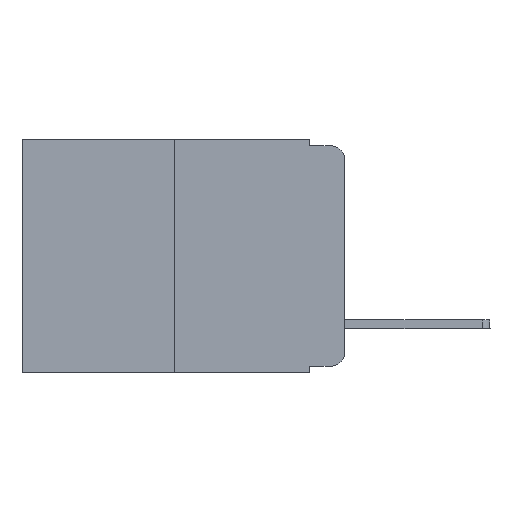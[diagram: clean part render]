
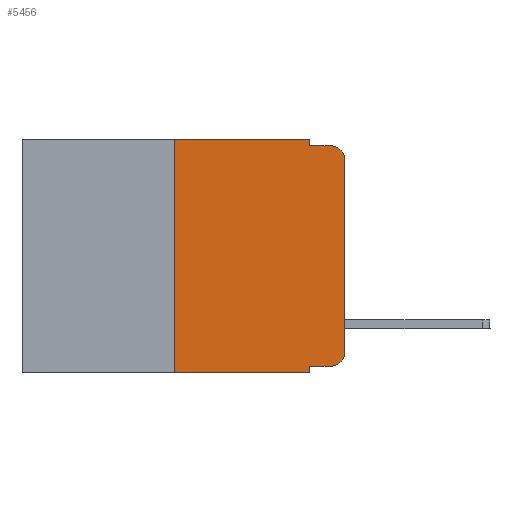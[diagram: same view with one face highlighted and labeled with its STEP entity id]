
A CAD part, left-side view. The second image highlights one B-rep face of the part: STEP entity #5456.
In plain terms, the highlighted planar face has unit normal (-1, 0, 0).
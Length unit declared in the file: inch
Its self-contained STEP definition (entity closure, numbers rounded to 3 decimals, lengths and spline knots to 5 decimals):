
#315 = CIRCLE ( 'NONE', #18076, 0.02 ) ;
#862 = CARTESIAN_POINT ( 'NONE',  ( 0., 0.473, 0. ) ) ;
#989 = DIRECTION ( 'NONE',  ( 0., -1., 0. ) ) ;
#1194 = LINE ( 'NONE', #10597, #11371 ) ;
#1485 = CARTESIAN_POINT ( 'NONE',  ( 0., 0.051, -0.333 ) ) ;
#1515 = DIRECTION ( 'NONE',  ( 0., 0., -1. ) ) ;
#1546 = VERTEX_POINT ( 'NONE', #13739 ) ;
#1560 = EDGE_CURVE ( 'NONE', #16669, #8262, #315, .T. ) ;
#1661 = VECTOR ( 'NONE', #1515, 39.37008 ) ;
#2155 = DIRECTION ( 'NONE',  ( 0., 0., -1. ) ) ;
#2189 = LINE ( 'NONE', #8463, #17527 ) ;
#2337 = DIRECTION ( 'NONE',  ( 0., 0., 1. ) ) ;
#2345 = EDGE_CURVE ( 'NONE', #1546, #4240, #16555, .T. ) ;
#2663 = EDGE_CURVE ( 'NONE', #6638, #1546, #8502, .T. ) ;
#3662 = CARTESIAN_POINT ( 'NONE',  ( 0., 0.25, 0. ) ) ;
#3822 = VECTOR ( 'NONE', #6338, 39.37008 ) ;
#3948 = ORIENTED_EDGE ( 'NONE', *, *, #2663, .F. ) ;
#4146 = EDGE_CURVE ( 'NONE', #17577, #16669, #2189, .T. ) ;
#4240 = VERTEX_POINT ( 'NONE', #6729 ) ;
#4476 = ORIENTED_EDGE ( 'NONE', *, *, #2345, .F. ) ;
#4644 = DIRECTION ( 'NONE',  ( 0., 0., 1. ) ) ;
#4836 = CARTESIAN_POINT ( 'NONE',  ( 0., 0.02, -0.01 ) ) ;
#4840 = CARTESIAN_POINT ( 'NONE',  ( 0., 0.473, 0. ) ) ;
#5456 = ADVANCED_FACE ( 'NONE', ( #16043 ), #9878, .F. ) ;
#5528 = LINE ( 'NONE', #3662, #7633 ) ;
#5599 = LINE ( 'NONE', #14200, #12645 ) ;
#5981 = CARTESIAN_POINT ( 'NONE',  ( 0., 0.051, 0. ) ) ;
#6224 = ORIENTED_EDGE ( 'NONE', *, *, #1560, .T. ) ;
#6271 = VERTEX_POINT ( 'NONE', #4836 ) ;
#6338 = DIRECTION ( 'NONE',  ( 0., -1., 0. ) ) ;
#6380 = CARTESIAN_POINT ( 'NONE',  ( 0., 0.051, -0.01 ) ) ;
#6416 = ORIENTED_EDGE ( 'NONE', *, *, #13997, .F. ) ;
#6638 = VERTEX_POINT ( 'NONE', #11368 ) ;
#6729 = CARTESIAN_POINT ( 'NONE',  ( 0., 0.051, -0.01 ) ) ;
#6916 = ORIENTED_EDGE ( 'NONE', *, *, #14733, .T. ) ;
#7131 = AXIS2_PLACEMENT_3D ( 'NONE', #862, #8509, #12958 ) ;
#7633 = VECTOR ( 'NONE', #2337, 39.37008 ) ;
#7795 = ORIENTED_EDGE ( 'NONE', *, *, #16438, .F. ) ;
#8019 = DIRECTION ( 'NONE',  ( -1., 0., 0. ) ) ;
#8103 = VERTEX_POINT ( 'NONE', #12424 ) ;
#8156 = CARTESIAN_POINT ( 'NONE',  ( 0., 0.02, -0.03 ) ) ;
#8262 = VERTEX_POINT ( 'NONE', #16104 ) ;
#8365 = LINE ( 'NONE', #6380, #18997 ) ;
#8463 = CARTESIAN_POINT ( 'NONE',  ( 0., 0.051, -0.333 ) ) ;
#8502 = LINE ( 'NONE', #4840, #3822 ) ;
#8509 = DIRECTION ( 'NONE',  ( 1., 0., 0. ) ) ;
#8674 = ORIENTED_EDGE ( 'NONE', *, *, #15822, .F. ) ;
#9121 = CARTESIAN_POINT ( 'NONE',  ( 0., 0.051, -0.343 ) ) ;
#9541 = VECTOR ( 'NONE', #989, 39.37008 ) ;
#9673 = AXIS2_PLACEMENT_3D ( 'NONE', #8156, #8019, #2155 ) ;
#9878 = PLANE ( 'NONE',  #7131 ) ;
#10597 = CARTESIAN_POINT ( 'NONE',  ( 0., 0., 0. ) ) ;
#10675 = DIRECTION ( 'NONE',  ( -1., 0., 0. ) ) ;
#10779 = EDGE_CURVE ( 'NONE', #8103, #6271, #11742, .T. ) ;
#11368 = CARTESIAN_POINT ( 'NONE',  ( 0., 0.25, 0. ) ) ;
#11371 = VECTOR ( 'NONE', #4644, 39.37008 ) ;
#11389 = CARTESIAN_POINT ( 'NONE',  ( 0., 0.02, -0.333 ) ) ;
#11742 = CIRCLE ( 'NONE', #9673, 0.02 ) ;
#11764 = EDGE_CURVE ( 'NONE', #17729, #12233, #15708, .T. ) ;
#11970 = DIRECTION ( 'NONE',  ( 0., -1., 0. ) ) ;
#12233 = VERTEX_POINT ( 'NONE', #9121 ) ;
#12424 = CARTESIAN_POINT ( 'NONE',  ( 0., 0., -0.03 ) ) ;
#12645 = VECTOR ( 'NONE', #14275, 39.37008 ) ;
#12958 = DIRECTION ( 'NONE',  ( 0., 0., -1. ) ) ;
#13549 = DIRECTION ( 'NONE',  ( 0., 0., -1. ) ) ;
#13739 = CARTESIAN_POINT ( 'NONE',  ( 0., 0.051, 0. ) ) ;
#13808 = CARTESIAN_POINT ( 'NONE',  ( 0., 0.02, -0.313 ) ) ;
#13990 = CARTESIAN_POINT ( 'NONE',  ( 0., 0.25, -0.343 ) ) ;
#13997 = EDGE_CURVE ( 'NONE', #17729, #6638, #5528, .T. ) ;
#14083 = EDGE_LOOP ( 'NONE', ( #6916, #14527, #7795, #4476, #3948, #6416, #17802, #8674, #16694, #6224 ) ) ;
#14200 = CARTESIAN_POINT ( 'NONE',  ( 0., 0.051, 0. ) ) ;
#14275 = DIRECTION ( 'NONE',  ( 0., 0., -1. ) ) ;
#14451 = DIRECTION ( 'NONE',  ( 0., -1., 0. ) ) ;
#14527 = ORIENTED_EDGE ( 'NONE', *, *, #10779, .T. ) ;
#14733 = EDGE_CURVE ( 'NONE', #8262, #8103, #1194, .T. ) ;
#15708 = LINE ( 'NONE', #16230, #9541 ) ;
#15822 = EDGE_CURVE ( 'NONE', #17577, #12233, #5599, .T. ) ;
#16043 = FACE_OUTER_BOUND ( 'NONE', #14083, .T. ) ;
#16104 = CARTESIAN_POINT ( 'NONE',  ( 0., 0., -0.313 ) ) ;
#16230 = CARTESIAN_POINT ( 'NONE',  ( 0., 0.473, -0.343 ) ) ;
#16438 = EDGE_CURVE ( 'NONE', #4240, #6271, #8365, .T. ) ;
#16555 = LINE ( 'NONE', #5981, #1661 ) ;
#16669 = VERTEX_POINT ( 'NONE', #11389 ) ;
#16694 = ORIENTED_EDGE ( 'NONE', *, *, #4146, .T. ) ;
#17527 = VECTOR ( 'NONE', #14451, 39.37008 ) ;
#17577 = VERTEX_POINT ( 'NONE', #1485 ) ;
#17729 = VERTEX_POINT ( 'NONE', #13990 ) ;
#17802 = ORIENTED_EDGE ( 'NONE', *, *, #11764, .T. ) ;
#18076 = AXIS2_PLACEMENT_3D ( 'NONE', #13808, #10675, #13549 ) ;
#18997 = VECTOR ( 'NONE', #11970, 39.37008 ) ;
